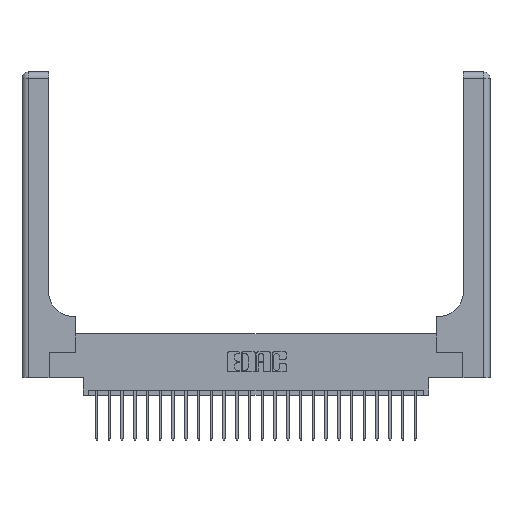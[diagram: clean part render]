
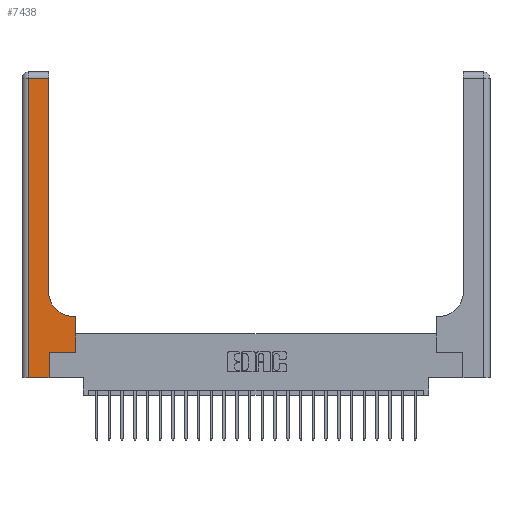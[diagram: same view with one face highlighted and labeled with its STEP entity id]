
A CAD part, top view. The second image highlights one B-rep face of the part: STEP entity #7438.
In plain terms, the highlighted planar face has unit normal (0, 0, 1).
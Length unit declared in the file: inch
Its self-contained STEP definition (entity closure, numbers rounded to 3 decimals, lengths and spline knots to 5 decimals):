
#76 = LINE ( 'NONE', #17370, #13973 ) ;
#1259 = CIRCLE ( 'NONE', #14979, 0.25 ) ;
#1476 = EDGE_CURVE ( 'NONE', #12072, #14192, #20471, .T. ) ;
#1695 = DIRECTION ( 'NONE',  ( 0., 1., 0. ) ) ;
#1768 = ORIENTED_EDGE ( 'NONE', *, *, #22377, .T. ) ;
#2221 = VECTOR ( 'NONE', #1695, 39.37008 ) ;
#2274 = VERTEX_POINT ( 'NONE', #22258 ) ;
#2649 = ORIENTED_EDGE ( 'NONE', *, *, #7917, .T. ) ;
#2893 = DIRECTION ( 'NONE',  ( 0., 0., -1. ) ) ;
#3147 = DIRECTION ( 'NONE',  ( -1., 0., 0. ) ) ;
#3339 = LINE ( 'NONE', #16990, #18374 ) ;
#3433 = DIRECTION ( 'NONE',  ( 0., 1., 0. ) ) ;
#4538 = CARTESIAN_POINT ( 'NONE',  ( 0., 3., 0.37 ) ) ;
#5206 = CARTESIAN_POINT ( 'NONE',  ( 0.265, 0., 0.37 ) ) ;
#5605 = CARTESIAN_POINT ( 'NONE',  ( 0.51, 0.6, 0.37 ) ) ;
#5722 = ORIENTED_EDGE ( 'NONE', *, *, #1476, .T. ) ;
#5912 = VERTEX_POINT ( 'NONE', #24123 ) ;
#6113 = ORIENTED_EDGE ( 'NONE', *, *, #22225, .T. ) ;
#6133 = VECTOR ( 'NONE', #10327, 39.37008 ) ;
#6192 = PLANE ( 'NONE',  #17111 ) ;
#6657 = LINE ( 'NONE', #14371, #6133 ) ;
#6747 = VECTOR ( 'NONE', #21540, 39.37008 ) ;
#7438 = ADVANCED_FACE ( 'NONE', ( #20179 ), #6192, .F. ) ;
#7507 = EDGE_CURVE ( 'NONE', #8705, #5912, #16547, .T. ) ;
#7837 = ORIENTED_EDGE ( 'NONE', *, *, #11712, .T. ) ;
#7917 = EDGE_CURVE ( 'NONE', #5912, #16750, #6657, .T. ) ;
#7976 = VECTOR ( 'NONE', #3433, 39.37008 ) ;
#8675 = CARTESIAN_POINT ( 'NONE',  ( 0.265, 0.25, 0.37 ) ) ;
#8705 = VERTEX_POINT ( 'NONE', #17580 ) ;
#9005 = LINE ( 'NONE', #16724, #2221 ) ;
#9069 = CARTESIAN_POINT ( 'NONE',  ( 0., 0., 0.37 ) ) ;
#9081 = CARTESIAN_POINT ( 'NONE',  ( 0., 2.94, 0.37 ) ) ;
#9648 = EDGE_LOOP ( 'NONE', ( #16676, #24090, #2649, #7837, #5722, #1768, #19846, #6113, #23075 ) ) ;
#10327 = DIRECTION ( 'NONE',  ( 0., -1., 0. ) ) ;
#10753 = CARTESIAN_POINT ( 'NONE',  ( 0.528, 0.25, 0.37 ) ) ;
#10834 = VERTEX_POINT ( 'NONE', #11779 ) ;
#11048 = DIRECTION ( 'NONE',  ( -1., 0., 0. ) ) ;
#11704 = CARTESIAN_POINT ( 'NONE',  ( 0.06, 0., 0.37 ) ) ;
#11712 = EDGE_CURVE ( 'NONE', #16750, #12072, #18657, .T. ) ;
#11779 = CARTESIAN_POINT ( 'NONE',  ( 0.528, 0.25, 0.37 ) ) ;
#12072 = VERTEX_POINT ( 'NONE', #24891 ) ;
#12765 = DIRECTION ( 'NONE',  ( 0., 1., 0. ) ) ;
#13248 = CARTESIAN_POINT ( 'NONE',  ( 0.51, 0.85, 0.37 ) ) ;
#13973 = VECTOR ( 'NONE', #15834, 39.37008 ) ;
#14148 = DIRECTION ( 'NONE',  ( -1., 0., 0. ) ) ;
#14176 = VERTEX_POINT ( 'NONE', #22408 ) ;
#14192 = VERTEX_POINT ( 'NONE', #8675 ) ;
#14371 = CARTESIAN_POINT ( 'NONE',  ( 0.06, 3., 0.37 ) ) ;
#14979 = AXIS2_PLACEMENT_3D ( 'NONE', #13248, #23068, #17176 ) ;
#15025 = EDGE_CURVE ( 'NONE', #15915, #2274, #1259, .T. ) ;
#15834 = DIRECTION ( 'NONE',  ( 1., 0., 0. ) ) ;
#15915 = VERTEX_POINT ( 'NONE', #5605 ) ;
#16547 = LINE ( 'NONE', #9081, #16716 ) ;
#16676 = ORIENTED_EDGE ( 'NONE', *, *, #20878, .T. ) ;
#16716 = VECTOR ( 'NONE', #3147, 39.37008 ) ;
#16724 = CARTESIAN_POINT ( 'NONE',  ( 0.26, 3., 0.37 ) ) ;
#16750 = VERTEX_POINT ( 'NONE', #11704 ) ;
#16990 = CARTESIAN_POINT ( 'NONE',  ( 0.26, 0.6, 0.37 ) ) ;
#17111 = AXIS2_PLACEMENT_3D ( 'NONE', #4538, #2893, #14148 ) ;
#17148 = VECTOR ( 'NONE', #12765, 39.37008 ) ;
#17176 = DIRECTION ( 'NONE',  ( 1., 0., 0. ) ) ;
#17370 = CARTESIAN_POINT ( 'NONE',  ( 0.265, 0.25, 0.37 ) ) ;
#17580 = CARTESIAN_POINT ( 'NONE',  ( 0.26, 2.94, 0.37 ) ) ;
#18320 = LINE ( 'NONE', #10753, #17148 ) ;
#18374 = VECTOR ( 'NONE', #11048, 39.37008 ) ;
#18657 = LINE ( 'NONE', #9069, #6747 ) ;
#19293 = EDGE_CURVE ( 'NONE', #10834, #14176, #18320, .T. ) ;
#19846 = ORIENTED_EDGE ( 'NONE', *, *, #19293, .T. ) ;
#20179 = FACE_OUTER_BOUND ( 'NONE', #9648, .T. ) ;
#20471 = LINE ( 'NONE', #5206, #7976 ) ;
#20878 = EDGE_CURVE ( 'NONE', #2274, #8705, #9005, .T. ) ;
#21540 = DIRECTION ( 'NONE',  ( 1., 0., 0. ) ) ;
#22225 = EDGE_CURVE ( 'NONE', #14176, #15915, #3339, .T. ) ;
#22258 = CARTESIAN_POINT ( 'NONE',  ( 0.26, 0.85, 0.37 ) ) ;
#22377 = EDGE_CURVE ( 'NONE', #14192, #10834, #76, .T. ) ;
#22408 = CARTESIAN_POINT ( 'NONE',  ( 0.528, 0.6, 0.37 ) ) ;
#23068 = DIRECTION ( 'NONE',  ( 0., 0., -1. ) ) ;
#23075 = ORIENTED_EDGE ( 'NONE', *, *, #15025, .T. ) ;
#24090 = ORIENTED_EDGE ( 'NONE', *, *, #7507, .T. ) ;
#24123 = CARTESIAN_POINT ( 'NONE',  ( 0.06, 2.94, 0.37 ) ) ;
#24891 = CARTESIAN_POINT ( 'NONE',  ( 0.265, 0., 0.37 ) ) ;
